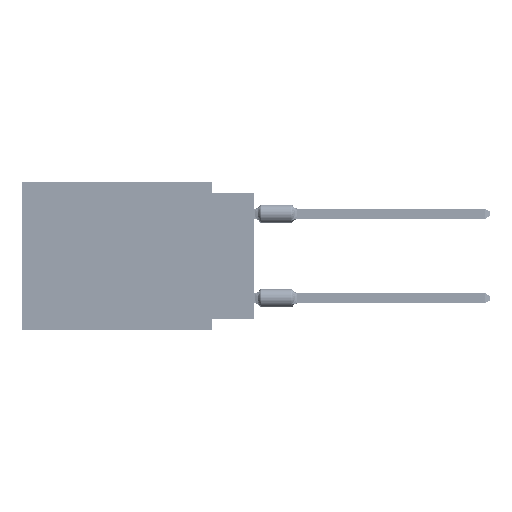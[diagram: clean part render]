
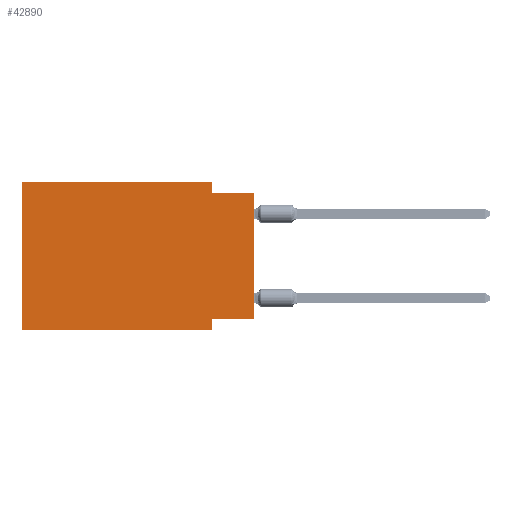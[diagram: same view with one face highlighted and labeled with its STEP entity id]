
A CAD part, left-side view. The second image highlights one B-rep face of the part: STEP entity #42890.
In plain terms, the highlighted planar face has unit normal (-1, 0, 0).
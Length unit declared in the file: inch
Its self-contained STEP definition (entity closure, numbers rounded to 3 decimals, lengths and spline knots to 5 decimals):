
#371 = DIRECTION ( 'NONE',  ( 0., 0., 1. ) ) ;
#1041 = VERTEX_POINT ( 'NONE', #65481 ) ;
#2880 = ORIENTED_EDGE ( 'NONE', *, *, #30786, .F. ) ;
#4368 = EDGE_CURVE ( 'NONE', #68698, #4608, #54910, .T. ) ;
#4608 = VERTEX_POINT ( 'NONE', #21990 ) ;
#6949 = DIRECTION ( 'NONE',  ( 0., 0., -1. ) ) ;
#7182 = CARTESIAN_POINT ( 'NONE',  ( 0., 0.1, -0.35 ) ) ;
#7423 = DIRECTION ( 'NONE',  ( 0., 1., 0. ) ) ;
#7956 = CARTESIAN_POINT ( 'NONE',  ( 0., 0.55, -0.35 ) ) ;
#9762 = ORIENTED_EDGE ( 'NONE', *, *, #44990, .F. ) ;
#11891 = LINE ( 'NONE', #58840, #14424 ) ;
#14424 = VECTOR ( 'NONE', #81825, 39.37008 ) ;
#18100 = LINE ( 'NONE', #49932, #47312 ) ;
#18834 = VECTOR ( 'NONE', #90507, 39.37008 ) ;
#20798 = VECTOR ( 'NONE', #43697, 39.37008 ) ;
#21990 = CARTESIAN_POINT ( 'NONE',  ( 0., 0.1, -0.325 ) ) ;
#23360 = LINE ( 'NONE', #7182, #71631 ) ;
#25661 = LINE ( 'NONE', #7956, #56350 ) ;
#26437 = ORIENTED_EDGE ( 'NONE', *, *, #52598, .T. ) ;
#26875 = LINE ( 'NONE', #58691, #18834 ) ;
#27194 = EDGE_CURVE ( 'NONE', #4608, #1041, #23360, .T. ) ;
#27526 = CARTESIAN_POINT ( 'NONE',  ( 0., 0.1, 0. ) ) ;
#30786 = EDGE_CURVE ( 'NONE', #40010, #35723, #11891, .T. ) ;
#35723 = VERTEX_POINT ( 'NONE', #89282 ) ;
#40010 = VERTEX_POINT ( 'NONE', #41128 ) ;
#40278 = CARTESIAN_POINT ( 'NONE',  ( 0., 0., -0.325 ) ) ;
#41128 = CARTESIAN_POINT ( 'NONE',  ( 0., 0.1, -0.025 ) ) ;
#41586 = DIRECTION ( 'NONE',  ( 0., 0., 1. ) ) ;
#42890 = ADVANCED_FACE ( 'NONE', ( #79991 ), #56494, .F. ) ;
#43697 = DIRECTION ( 'NONE',  ( 0., 0., -1. ) ) ;
#44990 = EDGE_CURVE ( 'NONE', #78549, #90894, #26875, .T. ) ;
#47312 = VECTOR ( 'NONE', #41586, 39.37008 ) ;
#49190 = ORIENTED_EDGE ( 'NONE', *, *, #92968, .F. ) ;
#49932 = CARTESIAN_POINT ( 'NONE',  ( 0., 0., 0. ) ) ;
#52572 = LINE ( 'NONE', #27526, #20798 ) ;
#52598 = EDGE_CURVE ( 'NONE', #95667, #1041, #25661, .T. ) ;
#53422 = EDGE_CURVE ( 'NONE', #95667, #78549, #94329, .T. ) ;
#54910 = LINE ( 'NONE', #78894, #69307 ) ;
#55947 = DIRECTION ( 'NONE',  ( 0., -1., 0. ) ) ;
#56350 = VECTOR ( 'NONE', #55947, 39.37008 ) ;
#56494 = PLANE ( 'NONE',  #93947 ) ;
#57265 = CARTESIAN_POINT ( 'NONE',  ( 0., 0.55, -0.35 ) ) ;
#58529 = EDGE_CURVE ( 'NONE', #68698, #35723, #18100, .T. ) ;
#58691 = CARTESIAN_POINT ( 'NONE',  ( 0., 0.55, 0. ) ) ;
#58840 = CARTESIAN_POINT ( 'NONE',  ( 0., 0., -0.025 ) ) ;
#62784 = DIRECTION ( 'NONE',  ( 1., 0., 0. ) ) ;
#62963 = ORIENTED_EDGE ( 'NONE', *, *, #58529, .T. ) ;
#63485 = CARTESIAN_POINT ( 'NONE',  ( 0., 0.1, 0. ) ) ;
#65481 = CARTESIAN_POINT ( 'NONE',  ( 0., 0.1, -0.35 ) ) ;
#68113 = VECTOR ( 'NONE', #371, 39.37008 ) ;
#68698 = VERTEX_POINT ( 'NONE', #40278 ) ;
#69307 = VECTOR ( 'NONE', #7423, 39.37008 ) ;
#71631 = VECTOR ( 'NONE', #94342, 39.37008 ) ;
#78549 = VERTEX_POINT ( 'NONE', #80837 ) ;
#78894 = CARTESIAN_POINT ( 'NONE',  ( 0., 0., -0.325 ) ) ;
#79046 = ORIENTED_EDGE ( 'NONE', *, *, #27194, .F. ) ;
#79991 = FACE_OUTER_BOUND ( 'NONE', #87687, .T. ) ;
#80837 = CARTESIAN_POINT ( 'NONE',  ( 0., 0.55, 0. ) ) ;
#80921 = ORIENTED_EDGE ( 'NONE', *, *, #4368, .F. ) ;
#81825 = DIRECTION ( 'NONE',  ( 0., -1., 0. ) ) ;
#85154 = ORIENTED_EDGE ( 'NONE', *, *, #53422, .F. ) ;
#87687 = EDGE_LOOP ( 'NONE', ( #62963, #2880, #49190, #9762, #85154, #26437, #79046, #80921 ) ) ;
#89282 = CARTESIAN_POINT ( 'NONE',  ( 0., 0., -0.025 ) ) ;
#90507 = DIRECTION ( 'NONE',  ( 0., -1., 0. ) ) ;
#90894 = VERTEX_POINT ( 'NONE', #63485 ) ;
#92968 = EDGE_CURVE ( 'NONE', #90894, #40010, #52572, .T. ) ;
#93947 = AXIS2_PLACEMENT_3D ( 'NONE', #94105, #62784, #6949 ) ;
#94105 = CARTESIAN_POINT ( 'NONE',  ( 0., 0.55, 0. ) ) ;
#94329 = LINE ( 'NONE', #102153, #68113 ) ;
#94342 = DIRECTION ( 'NONE',  ( 0., 0., -1. ) ) ;
#95667 = VERTEX_POINT ( 'NONE', #57265 ) ;
#102153 = CARTESIAN_POINT ( 'NONE',  ( 0., 0.55, 0. ) ) ;
